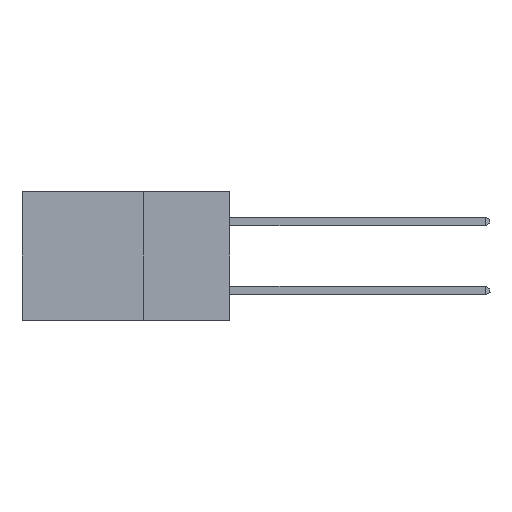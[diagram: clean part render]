
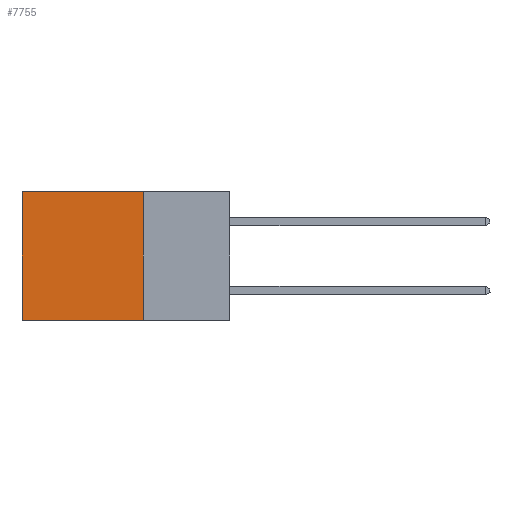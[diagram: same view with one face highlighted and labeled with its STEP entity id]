
A CAD part, left-side view. The second image highlights one B-rep face of the part: STEP entity #7755.
In plain terms, the highlighted planar face has unit normal (-1, 0, 0).
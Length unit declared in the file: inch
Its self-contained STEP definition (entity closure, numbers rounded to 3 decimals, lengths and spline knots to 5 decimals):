
#357 = LINE ( 'NONE', #2284, #6758 ) ;
#554 = DIRECTION ( 'NONE',  ( 0., 0., -1. ) ) ;
#563 = CARTESIAN_POINT ( 'NONE',  ( 0.298, 0.6, 0. ) ) ;
#1272 = ORIENTED_EDGE ( 'NONE', *, *, #4940, .F. ) ;
#1515 = VERTEX_POINT ( 'NONE', #3410 ) ;
#2284 = CARTESIAN_POINT ( 'NONE',  ( 0.298, 0.25, 0. ) ) ;
#2366 = CARTESIAN_POINT ( 'NONE',  ( 0.298, 0.25, 0. ) ) ;
#2507 = CARTESIAN_POINT ( 'NONE',  ( 0.298, 0.25, -0.37 ) ) ;
#2659 = ORIENTED_EDGE ( 'NONE', *, *, #9218, .T. ) ;
#2667 = EDGE_CURVE ( 'NONE', #1515, #5202, #3030, .T. ) ;
#3030 = LINE ( 'NONE', #563, #5878 ) ;
#3410 = CARTESIAN_POINT ( 'NONE',  ( 0.298, 0.6, 0. ) ) ;
#3891 = CARTESIAN_POINT ( 'NONE',  ( 0.298, 0.6, -0.37 ) ) ;
#3987 = VECTOR ( 'NONE', #5945, 39.37008 ) ;
#4454 = DIRECTION ( 'NONE',  ( 1., 0., 0. ) ) ;
#4461 = VECTOR ( 'NONE', #554, 39.37008 ) ;
#4542 = PLANE ( 'NONE',  #9788 ) ;
#4628 = EDGE_LOOP ( 'NONE', ( #10003, #9569, #1272, #2659 ) ) ;
#4940 = EDGE_CURVE ( 'NONE', #6716, #7220, #7597, .T. ) ;
#5202 = VERTEX_POINT ( 'NONE', #3891 ) ;
#5768 = LINE ( 'NONE', #5918, #3987 ) ;
#5878 = VECTOR ( 'NONE', #7175, 39.37008 ) ;
#5918 = CARTESIAN_POINT ( 'NONE',  ( 0.298, 0.25, -0.37 ) ) ;
#5945 = DIRECTION ( 'NONE',  ( 0., 1., 0. ) ) ;
#6450 = EDGE_CURVE ( 'NONE', #7220, #5202, #5768, .T. ) ;
#6511 = CARTESIAN_POINT ( 'NONE',  ( 0.298, 0.25, 0. ) ) ;
#6647 = FACE_OUTER_BOUND ( 'NONE', #4628, .T. ) ;
#6716 = VERTEX_POINT ( 'NONE', #2366 ) ;
#6758 = VECTOR ( 'NONE', #6931, 39.37008 ) ;
#6931 = DIRECTION ( 'NONE',  ( 0., 1., 0. ) ) ;
#7175 = DIRECTION ( 'NONE',  ( 0., 0., -1. ) ) ;
#7220 = VERTEX_POINT ( 'NONE', #2507 ) ;
#7597 = LINE ( 'NONE', #10001, #4461 ) ;
#7755 = ADVANCED_FACE ( 'NONE', ( #6647 ), #4542, .F. ) ;
#9218 = EDGE_CURVE ( 'NONE', #6716, #1515, #357, .T. ) ;
#9569 = ORIENTED_EDGE ( 'NONE', *, *, #6450, .F. ) ;
#9788 = AXIS2_PLACEMENT_3D ( 'NONE', #6511, #4454, #12161 ) ;
#10001 = CARTESIAN_POINT ( 'NONE',  ( 0.298, 0.25, 0. ) ) ;
#10003 = ORIENTED_EDGE ( 'NONE', *, *, #2667, .T. ) ;
#12161 = DIRECTION ( 'NONE',  ( 0., 0., -1. ) ) ;
